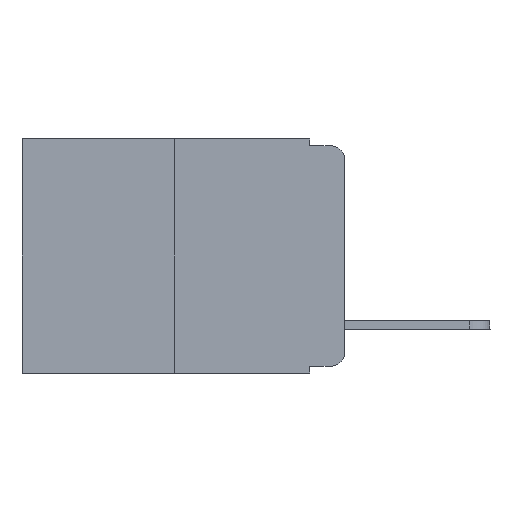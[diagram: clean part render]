
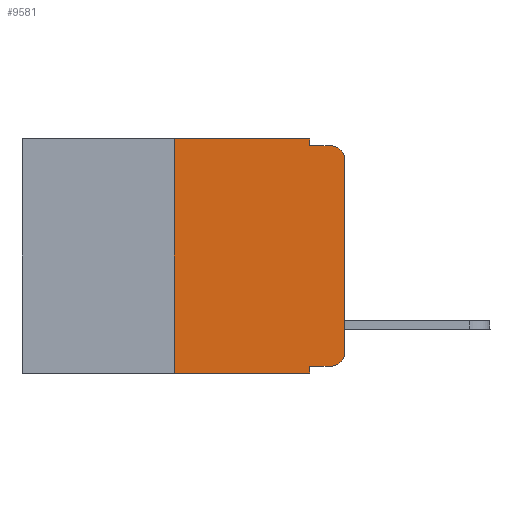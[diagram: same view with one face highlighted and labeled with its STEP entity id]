
A CAD part, left-side view. The second image highlights one B-rep face of the part: STEP entity #9581.
In plain terms, the highlighted planar face has unit normal (-1, 0, 0).
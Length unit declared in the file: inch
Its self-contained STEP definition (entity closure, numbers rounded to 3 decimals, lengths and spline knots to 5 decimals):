
#901 = EDGE_CURVE ( 'NONE', #22279, #5780, #16213, .T. ) ;
#902 = DIRECTION ( 'NONE',  ( 0., -1., 0. ) ) ;
#1102 = VERTEX_POINT ( 'NONE', #1567 ) ;
#1260 = CARTESIAN_POINT ( 'NONE',  ( 0., 0.02, -0.313 ) ) ;
#1567 = CARTESIAN_POINT ( 'NONE',  ( 0., 0.051, 0. ) ) ;
#1673 = AXIS2_PLACEMENT_3D ( 'NONE', #7645, #7877, #18567 ) ;
#2079 = EDGE_CURVE ( 'NONE', #1102, #18018, #17725, .T. ) ;
#2392 = VERTEX_POINT ( 'NONE', #21427 ) ;
#2663 = DIRECTION ( 'NONE',  ( 0., 0., -1. ) ) ;
#3001 = EDGE_CURVE ( 'NONE', #22279, #17150, #16400, .T. ) ;
#3068 = EDGE_CURVE ( 'NONE', #18365, #2392, #12724, .T. ) ;
#3073 = VECTOR ( 'NONE', #7195, 39.37008 ) ;
#3132 = ORIENTED_EDGE ( 'NONE', *, *, #14887, .F. ) ;
#3485 = AXIS2_PLACEMENT_3D ( 'NONE', #1260, #23026, #8322 ) ;
#3810 = CARTESIAN_POINT ( 'NONE',  ( 0., 0.051, -0.333 ) ) ;
#3875 = VECTOR ( 'NONE', #902, 39.37008 ) ;
#4105 = LINE ( 'NONE', #19953, #17703 ) ;
#4210 = CARTESIAN_POINT ( 'NONE',  ( 0., 0.051, 0. ) ) ;
#4489 = CARTESIAN_POINT ( 'NONE',  ( 0., 0.25, -0.343 ) ) ;
#4558 = CARTESIAN_POINT ( 'NONE',  ( 0., 0., -0.03 ) ) ;
#4918 = VERTEX_POINT ( 'NONE', #15253 ) ;
#4939 = VECTOR ( 'NONE', #7542, 39.37008 ) ;
#5580 = VECTOR ( 'NONE', #8911, 39.37008 ) ;
#5734 = DIRECTION ( 'NONE',  ( 0., -1., 0. ) ) ;
#5780 = VERTEX_POINT ( 'NONE', #15079 ) ;
#6247 = DIRECTION ( 'NONE',  ( 1., 0., 0. ) ) ;
#6662 = ORIENTED_EDGE ( 'NONE', *, *, #18336, .F. ) ;
#7013 = ORIENTED_EDGE ( 'NONE', *, *, #3068, .T. ) ;
#7171 = EDGE_CURVE ( 'NONE', #17150, #1102, #20573, .T. ) ;
#7195 = DIRECTION ( 'NONE',  ( 0., 0., 1. ) ) ;
#7542 = DIRECTION ( 'NONE',  ( 0., -1., 0. ) ) ;
#7645 = CARTESIAN_POINT ( 'NONE',  ( 0., 0.02, -0.03 ) ) ;
#7718 = CARTESIAN_POINT ( 'NONE',  ( 0., 0.473, -0.343 ) ) ;
#7877 = DIRECTION ( 'NONE',  ( -1., 0., 0. ) ) ;
#8014 = DIRECTION ( 'NONE',  ( 0., -1., 0. ) ) ;
#8205 = EDGE_CURVE ( 'NONE', #19780, #18999, #17463, .T. ) ;
#8322 = DIRECTION ( 'NONE',  ( 0., 0., -1. ) ) ;
#8690 = ORIENTED_EDGE ( 'NONE', *, *, #7171, .F. ) ;
#8911 = DIRECTION ( 'NONE',  ( 0., 0., -1. ) ) ;
#9374 = ORIENTED_EDGE ( 'NONE', *, *, #2079, .F. ) ;
#9390 = ORIENTED_EDGE ( 'NONE', *, *, #8205, .T. ) ;
#9403 = DIRECTION ( 'NONE',  ( 0., 0., -1. ) ) ;
#9581 = ADVANCED_FACE ( 'NONE', ( #18794 ), #14955, .F. ) ;
#9769 = CARTESIAN_POINT ( 'NONE',  ( 0., 0.473, 0. ) ) ;
#10585 = CARTESIAN_POINT ( 'NONE',  ( 0., 0.051, -0.01 ) ) ;
#10629 = VECTOR ( 'NONE', #5734, 39.37008 ) ;
#11070 = EDGE_CURVE ( 'NONE', #2392, #4918, #22984, .T. ) ;
#11867 = CARTESIAN_POINT ( 'NONE',  ( 0., 0.02, -0.01 ) ) ;
#12550 = AXIS2_PLACEMENT_3D ( 'NONE', #20657, #6247, #9403 ) ;
#12724 = LINE ( 'NONE', #3810, #4939 ) ;
#13095 = ORIENTED_EDGE ( 'NONE', *, *, #3001, .F. ) ;
#13611 = ORIENTED_EDGE ( 'NONE', *, *, #901, .T. ) ;
#13720 = CARTESIAN_POINT ( 'NONE',  ( 0., 0.25, 0. ) ) ;
#14887 = EDGE_CURVE ( 'NONE', #18365, #5780, #18527, .T. ) ;
#14955 = PLANE ( 'NONE',  #12550 ) ;
#15079 = CARTESIAN_POINT ( 'NONE',  ( 0., 0.051, -0.343 ) ) ;
#15253 = CARTESIAN_POINT ( 'NONE',  ( 0., 0., -0.313 ) ) ;
#15306 = LINE ( 'NONE', #17713, #3875 ) ;
#15715 = CARTESIAN_POINT ( 'NONE',  ( 0., 0.25, 0. ) ) ;
#15895 = VECTOR ( 'NONE', #8014, 39.37008 ) ;
#16213 = LINE ( 'NONE', #7718, #10629 ) ;
#16354 = DIRECTION ( 'NONE',  ( 0., 0., 1. ) ) ;
#16400 = LINE ( 'NONE', #15715, #3073 ) ;
#16576 = EDGE_LOOP ( 'NONE', ( #22988, #9390, #6662, #9374, #8690, #13095, #13611, #3132, #7013, #20256 ) ) ;
#16759 = EDGE_CURVE ( 'NONE', #4918, #19780, #4105, .T. ) ;
#17150 = VERTEX_POINT ( 'NONE', #13720 ) ;
#17463 = CIRCLE ( 'NONE', #1673, 0.02 ) ;
#17703 = VECTOR ( 'NONE', #16354, 39.37008 ) ;
#17713 = CARTESIAN_POINT ( 'NONE',  ( 0., 0.051, -0.01 ) ) ;
#17725 = LINE ( 'NONE', #21223, #5580 ) ;
#18018 = VERTEX_POINT ( 'NONE', #10585 ) ;
#18336 = EDGE_CURVE ( 'NONE', #18018, #18999, #15306, .T. ) ;
#18357 = VECTOR ( 'NONE', #2663, 39.37008 ) ;
#18365 = VERTEX_POINT ( 'NONE', #18797 ) ;
#18527 = LINE ( 'NONE', #4210, #18357 ) ;
#18567 = DIRECTION ( 'NONE',  ( 0., 0., -1. ) ) ;
#18794 = FACE_OUTER_BOUND ( 'NONE', #16576, .T. ) ;
#18797 = CARTESIAN_POINT ( 'NONE',  ( 0., 0.051, -0.333 ) ) ;
#18999 = VERTEX_POINT ( 'NONE', #11867 ) ;
#19780 = VERTEX_POINT ( 'NONE', #4558 ) ;
#19953 = CARTESIAN_POINT ( 'NONE',  ( 0., 0., 0. ) ) ;
#20256 = ORIENTED_EDGE ( 'NONE', *, *, #11070, .T. ) ;
#20573 = LINE ( 'NONE', #9769, #15895 ) ;
#20657 = CARTESIAN_POINT ( 'NONE',  ( 0., 0.473, 0. ) ) ;
#21223 = CARTESIAN_POINT ( 'NONE',  ( 0., 0.051, 0. ) ) ;
#21427 = CARTESIAN_POINT ( 'NONE',  ( 0., 0.02, -0.333 ) ) ;
#22279 = VERTEX_POINT ( 'NONE', #4489 ) ;
#22984 = CIRCLE ( 'NONE', #3485, 0.02 ) ;
#22988 = ORIENTED_EDGE ( 'NONE', *, *, #16759, .T. ) ;
#23026 = DIRECTION ( 'NONE',  ( -1., 0., 0. ) ) ;
